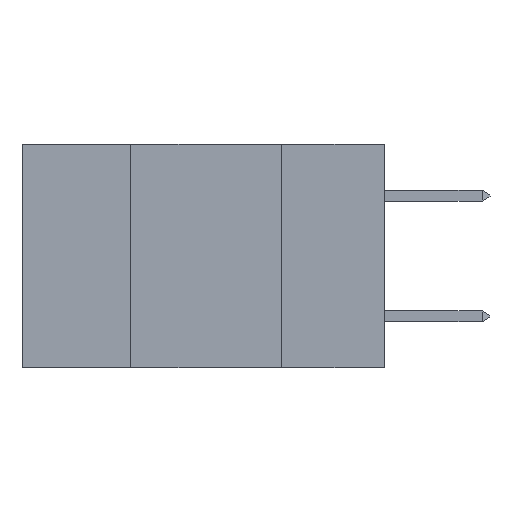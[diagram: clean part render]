
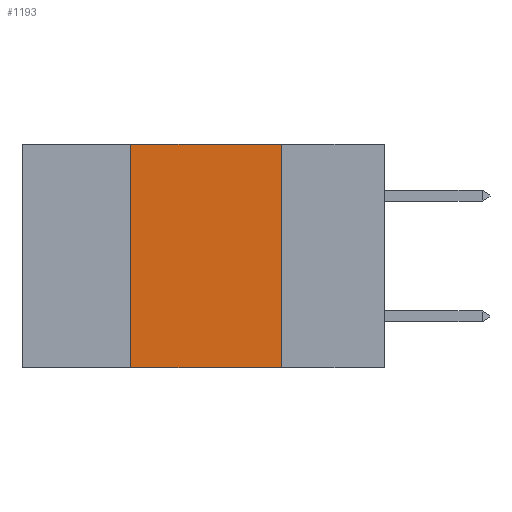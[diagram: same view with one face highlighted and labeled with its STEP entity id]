
A CAD part, left-side view. The second image highlights one B-rep face of the part: STEP entity #1193.
In plain terms, the highlighted planar face has unit normal (-1, 0, 0).
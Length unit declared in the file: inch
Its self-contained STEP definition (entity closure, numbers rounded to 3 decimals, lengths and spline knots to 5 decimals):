
#104 = VERTEX_POINT ( 'NONE', #5776 ) ;
#169 = EDGE_CURVE ( 'NONE', #10010, #1813, #4391, .T. ) ;
#180 = CARTESIAN_POINT ( 'NONE',  ( 0., 0.42, 0. ) ) ;
#332 = VERTEX_POINT ( 'NONE', #8521 ) ;
#682 = CARTESIAN_POINT ( 'NONE',  ( 0., 0.6, 0. ) ) ;
#1193 = ADVANCED_FACE ( 'NONE', ( #3078 ), #4470, .F. ) ;
#1498 = DIRECTION ( 'NONE',  ( 0., -1., 0. ) ) ;
#1712 = EDGE_LOOP ( 'NONE', ( #8937, #3656, #7745, #7250 ) ) ;
#1813 = VERTEX_POINT ( 'NONE', #6633 ) ;
#2288 = EDGE_CURVE ( 'NONE', #104, #332, #5715, .T. ) ;
#3078 = FACE_OUTER_BOUND ( 'NONE', #1712, .T. ) ;
#3221 = VECTOR ( 'NONE', #4658, 39.37008 ) ;
#3656 = ORIENTED_EDGE ( 'NONE', *, *, #169, .F. ) ;
#4095 = LINE ( 'NONE', #5625, #3221 ) ;
#4239 = VECTOR ( 'NONE', #1498, 39.37008 ) ;
#4391 = LINE ( 'NONE', #9915, #8130 ) ;
#4470 = PLANE ( 'NONE',  #4552 ) ;
#4552 = AXIS2_PLACEMENT_3D ( 'NONE', #682, #10001, #8556 ) ;
#4658 = DIRECTION ( 'NONE',  ( 0., 0., 1. ) ) ;
#4737 = EDGE_CURVE ( 'NONE', #104, #10010, #4095, .T. ) ;
#5425 = EDGE_CURVE ( 'NONE', #1813, #332, #6911, .T. ) ;
#5625 = CARTESIAN_POINT ( 'NONE',  ( 0., 0.42, 0. ) ) ;
#5715 = LINE ( 'NONE', #7031, #4239 ) ;
#5776 = CARTESIAN_POINT ( 'NONE',  ( 0., 0.42, -0.37 ) ) ;
#6119 = DIRECTION ( 'NONE',  ( 0., 0., -1. ) ) ;
#6633 = CARTESIAN_POINT ( 'NONE',  ( 0., 0.17, 0. ) ) ;
#6911 = LINE ( 'NONE', #9962, #9363 ) ;
#7031 = CARTESIAN_POINT ( 'NONE',  ( 0., 0.6, -0.37 ) ) ;
#7250 = ORIENTED_EDGE ( 'NONE', *, *, #2288, .T. ) ;
#7745 = ORIENTED_EDGE ( 'NONE', *, *, #4737, .F. ) ;
#8130 = VECTOR ( 'NONE', #9146, 39.37008 ) ;
#8521 = CARTESIAN_POINT ( 'NONE',  ( 0., 0.17, -0.37 ) ) ;
#8556 = DIRECTION ( 'NONE',  ( 0., 0., -1. ) ) ;
#8937 = ORIENTED_EDGE ( 'NONE', *, *, #5425, .F. ) ;
#9146 = DIRECTION ( 'NONE',  ( 0., -1., 0. ) ) ;
#9363 = VECTOR ( 'NONE', #6119, 39.37008 ) ;
#9915 = CARTESIAN_POINT ( 'NONE',  ( 0., 0.6, 0. ) ) ;
#9962 = CARTESIAN_POINT ( 'NONE',  ( 0., 0.17, 0. ) ) ;
#10001 = DIRECTION ( 'NONE',  ( 1., 0., 0. ) ) ;
#10010 = VERTEX_POINT ( 'NONE', #180 ) ;
